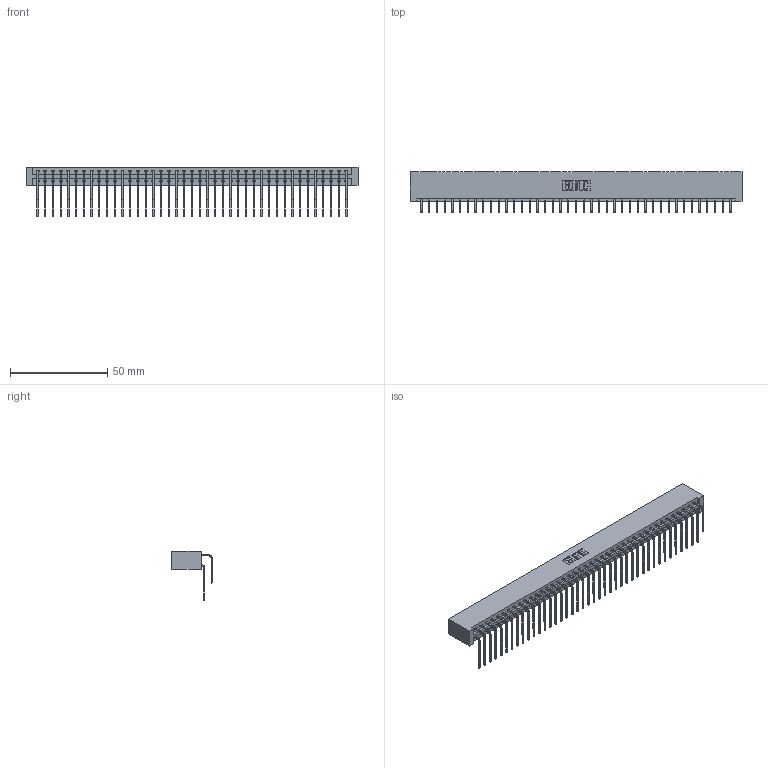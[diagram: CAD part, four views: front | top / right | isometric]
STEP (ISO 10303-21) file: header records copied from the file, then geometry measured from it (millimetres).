
FILE_DESCRIPTION (( 'STEP AP203' ), '1' );
FILE_NAME ('387-082-559-201.STEP', '2018-09-23T21:01:08', ( '' ), ( '' ), 'SwSTEP 2.0', 'SolidWorks 2016', '' );
FILE_SCHEMA (( 'CONFIG_CONTROL_DESIGN' ));
Length unit declared in the file: inch
Products named in the file (4): 345-292-001_558 559 Tail - 1; 345-292-001_559 Tail - 2; 387-082-559-201; 337 Part_No Mounting Lugs
Assembly tree (83 placements, depth 2):
  387-082-559-201
    337 Part_No Mounting Lugs
    345-292-001_558 559 Tail - 1  x41
    345-292-001_559 Tail - 2  x41
Bounding box: 170.33 x 20.9 x 25.53 mm (x, y, z)
Volume: 19171.4 mm3; surface area: 24095 mm2
Topology: 83 solids, 83 shells, 4698 faces, 13981 edges, 9210 vertices
Faces by surface type: plane 3346, cylinder 1352
Entity records: 33425 total; most frequent: CARTESIAN_POINT 5677, ORIENTED_EDGE 5562, DIRECTION 4805, EDGE_CURVE 2781, VECTOR 2621, LINE 2621, VERTEX_POINT 1850, AXIS2_PLACEMENT_3D 1092
